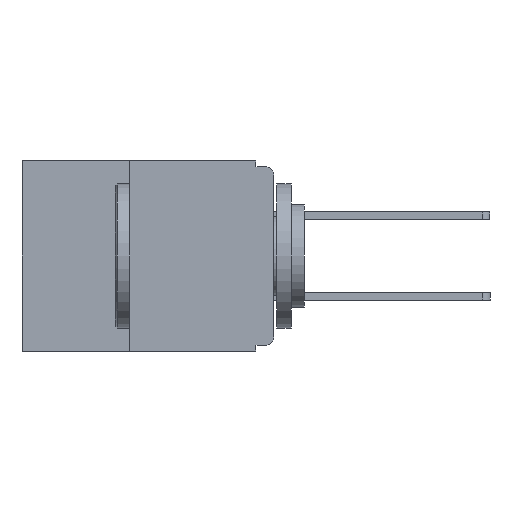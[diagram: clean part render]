
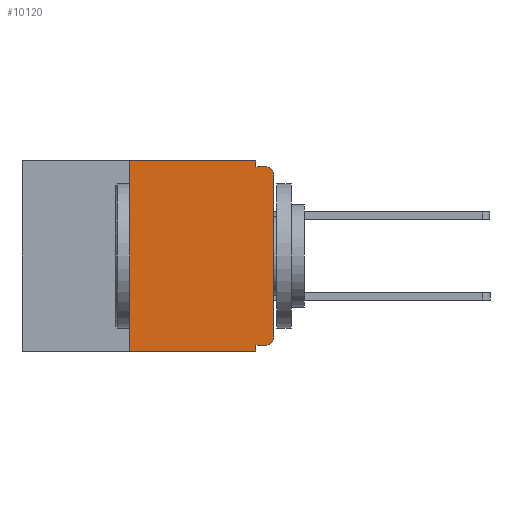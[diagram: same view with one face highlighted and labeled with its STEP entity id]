
A CAD part, left-side view. The second image highlights one B-rep face of the part: STEP entity #10120.
In plain terms, the highlighted planar face has unit normal (-1, 0, 0).
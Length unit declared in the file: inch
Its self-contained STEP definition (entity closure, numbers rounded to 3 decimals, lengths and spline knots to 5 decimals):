
#473 = VECTOR ( 'NONE', #10294, 39.37008 ) ;
#1450 = CIRCLE ( 'NONE', #11163, 0.015 ) ;
#2442 = VERTEX_POINT ( 'NONE', #12681 ) ;
#2490 = VERTEX_POINT ( 'NONE', #11914 ) ;
#2595 = VERTEX_POINT ( 'NONE', #9259 ) ;
#2613 = DIRECTION ( 'NONE',  ( 0., 0., -1. ) ) ;
#2636 = LINE ( 'NONE', #23756, #23169 ) ;
#2677 = VECTOR ( 'NONE', #21301, 39.37008 ) ;
#2992 = ORIENTED_EDGE ( 'NONE', *, *, #13732, .F. ) ;
#3308 = ORIENTED_EDGE ( 'NONE', *, *, #3858, .T. ) ;
#3539 = EDGE_CURVE ( 'NONE', #15682, #21411, #13754, .T. ) ;
#3806 = DIRECTION ( 'NONE',  ( 0., -1., 0. ) ) ;
#3858 = EDGE_CURVE ( 'NONE', #16402, #2442, #10998, .T. ) ;
#5394 = DIRECTION ( 'NONE',  ( 0., 0., -1. ) ) ;
#5767 = ORIENTED_EDGE ( 'NONE', *, *, #3539, .F. ) ;
#5937 = EDGE_CURVE ( 'NONE', #2442, #6294, #12390, .T. ) ;
#6271 = AXIS2_PLACEMENT_3D ( 'NONE', #18298, #6790, #20238 ) ;
#6294 = VERTEX_POINT ( 'NONE', #12058 ) ;
#6614 = DIRECTION ( 'NONE',  ( 0., 1., 0. ) ) ;
#6790 = DIRECTION ( 'NONE',  ( 1., 0., 0. ) ) ;
#7016 = ORIENTED_EDGE ( 'NONE', *, *, #15457, .T. ) ;
#7271 = CARTESIAN_POINT ( 'NONE',  ( 0., 0.031, 0. ) ) ;
#7852 = EDGE_CURVE ( 'NONE', #21411, #2595, #14973, .T. ) ;
#9154 = ORIENTED_EDGE ( 'NONE', *, *, #5937, .T. ) ;
#9259 = CARTESIAN_POINT ( 'NONE',  ( 0., 0.031, 0. ) ) ;
#9693 = AXIS2_PLACEMENT_3D ( 'NONE', #22452, #11036, #24278 ) ;
#9779 = ORIENTED_EDGE ( 'NONE', *, *, #13789, .F. ) ;
#10120 = ADVANCED_FACE ( 'NONE', ( #19618 ), #12539, .F. ) ;
#10294 = DIRECTION ( 'NONE',  ( 0., 0., 1. ) ) ;
#10661 = CARTESIAN_POINT ( 'NONE',  ( 0., 0., -0.01 ) ) ;
#10998 = LINE ( 'NONE', #12107, #473 ) ;
#11036 = DIRECTION ( 'NONE',  ( -1., 0., 0. ) ) ;
#11070 = VERTEX_POINT ( 'NONE', #12833 ) ;
#11131 = DIRECTION ( 'NONE',  ( -1., 0., 0. ) ) ;
#11163 = AXIS2_PLACEMENT_3D ( 'NONE', #22551, #11131, #24377 ) ;
#11656 = LINE ( 'NONE', #21578, #21175 ) ;
#11761 = VECTOR ( 'NONE', #6614, 39.37008 ) ;
#11914 = CARTESIAN_POINT ( 'NONE',  ( 0., 0.015, -0.32 ) ) ;
#12058 = CARTESIAN_POINT ( 'NONE',  ( 0., 0.015, -0.01 ) ) ;
#12107 = CARTESIAN_POINT ( 'NONE',  ( 0., 0., 0. ) ) ;
#12390 = CIRCLE ( 'NONE', #9693, 0.015 ) ;
#12539 = PLANE ( 'NONE',  #6271 ) ;
#12681 = CARTESIAN_POINT ( 'NONE',  ( 0., 0., -0.025 ) ) ;
#12833 = CARTESIAN_POINT ( 'NONE',  ( 0., 0.031, -0.01 ) ) ;
#12841 = ORIENTED_EDGE ( 'NONE', *, *, #18140, .F. ) ;
#12955 = LINE ( 'NONE', #7271, #13563 ) ;
#13563 = VECTOR ( 'NONE', #5394, 39.37008 ) ;
#13732 = EDGE_CURVE ( 'NONE', #2490, #13942, #16792, .T. ) ;
#13754 = LINE ( 'NONE', #23514, #2677 ) ;
#13789 = EDGE_CURVE ( 'NONE', #11070, #6294, #20657, .T. ) ;
#13792 = VECTOR ( 'NONE', #3806, 39.37008 ) ;
#13942 = VERTEX_POINT ( 'NONE', #22490 ) ;
#14560 = DIRECTION ( 'NONE',  ( 0., -1., 0. ) ) ;
#14923 = ORIENTED_EDGE ( 'NONE', *, *, #24395, .F. ) ;
#14973 = LINE ( 'NONE', #17322, #13792 ) ;
#15102 = EDGE_LOOP ( 'NONE', ( #3308, #9154, #9779, #14923, #20545, #5767, #7016, #12841, #2992, #24052 ) ) ;
#15457 = EDGE_CURVE ( 'NONE', #15682, #16283, #11656, .T. ) ;
#15616 = VECTOR ( 'NONE', #14560, 39.37008 ) ;
#15682 = VERTEX_POINT ( 'NONE', #22157 ) ;
#16274 = CARTESIAN_POINT ( 'NONE',  ( 0., 0., -0.32 ) ) ;
#16283 = VERTEX_POINT ( 'NONE', #20375 ) ;
#16402 = VERTEX_POINT ( 'NONE', #16948 ) ;
#16792 = LINE ( 'NONE', #16274, #11761 ) ;
#16948 = CARTESIAN_POINT ( 'NONE',  ( 0., 0., -0.305 ) ) ;
#17322 = CARTESIAN_POINT ( 'NONE',  ( 0., 0.437, 0. ) ) ;
#17811 = CARTESIAN_POINT ( 'NONE',  ( 0., 0.25, 0. ) ) ;
#18140 = EDGE_CURVE ( 'NONE', #13942, #16283, #2636, .T. ) ;
#18298 = CARTESIAN_POINT ( 'NONE',  ( 0., 0.437, 0. ) ) ;
#19618 = FACE_OUTER_BOUND ( 'NONE', #15102, .T. ) ;
#20238 = DIRECTION ( 'NONE',  ( 0., 0., -1. ) ) ;
#20375 = CARTESIAN_POINT ( 'NONE',  ( 0., 0.031, -0.33 ) ) ;
#20545 = ORIENTED_EDGE ( 'NONE', *, *, #7852, .F. ) ;
#20657 = LINE ( 'NONE', #10661, #15616 ) ;
#21175 = VECTOR ( 'NONE', #23442, 39.37008 ) ;
#21301 = DIRECTION ( 'NONE',  ( 0., 0., 1. ) ) ;
#21411 = VERTEX_POINT ( 'NONE', #17811 ) ;
#21578 = CARTESIAN_POINT ( 'NONE',  ( 0., 0.437, -0.33 ) ) ;
#22157 = CARTESIAN_POINT ( 'NONE',  ( 0., 0.25, -0.33 ) ) ;
#22452 = CARTESIAN_POINT ( 'NONE',  ( 0., 0.015, -0.025 ) ) ;
#22490 = CARTESIAN_POINT ( 'NONE',  ( 0., 0.031, -0.32 ) ) ;
#22551 = CARTESIAN_POINT ( 'NONE',  ( 0., 0.015, -0.305 ) ) ;
#22594 = EDGE_CURVE ( 'NONE', #2490, #16402, #1450, .T. ) ;
#23169 = VECTOR ( 'NONE', #2613, 39.37008 ) ;
#23442 = DIRECTION ( 'NONE',  ( 0., -1., 0. ) ) ;
#23514 = CARTESIAN_POINT ( 'NONE',  ( 0., 0.25, -0.33 ) ) ;
#23756 = CARTESIAN_POINT ( 'NONE',  ( 0., 0.031, -0.33 ) ) ;
#24052 = ORIENTED_EDGE ( 'NONE', *, *, #22594, .T. ) ;
#24278 = DIRECTION ( 'NONE',  ( 0., 0., -1. ) ) ;
#24377 = DIRECTION ( 'NONE',  ( 0., 0., -1. ) ) ;
#24395 = EDGE_CURVE ( 'NONE', #2595, #11070, #12955, .T. ) ;
